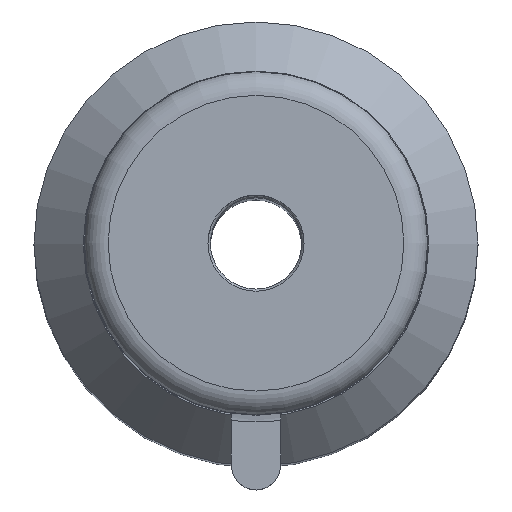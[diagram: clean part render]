
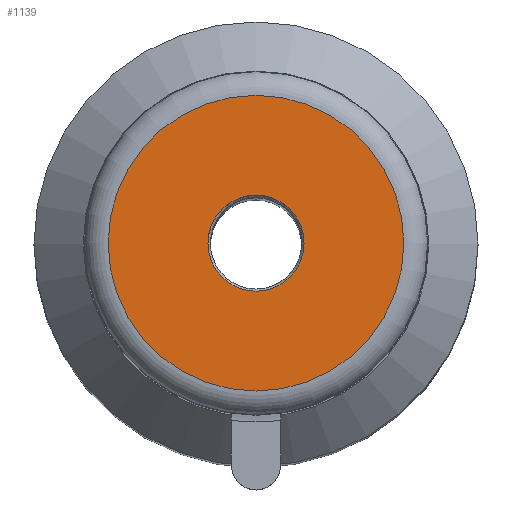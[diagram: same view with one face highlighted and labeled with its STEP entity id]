
A CAD part, top view. The second image highlights one B-rep face of the part: STEP entity #1139.
In plain terms, the highlighted planar face has unit normal (0, 0, 1).
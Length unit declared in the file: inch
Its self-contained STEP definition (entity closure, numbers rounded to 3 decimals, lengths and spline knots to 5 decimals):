
#926=CARTESIAN_POINT('',(-0.195,0.0,2.5));
#927=VERTEX_POINT('',#926);
#928=CARTESIAN_POINT('',(0.0,0.0,2.5));
#929=DIRECTION('',(0.0,0.0,-1.0));
#930=DIRECTION('',(-1.0,0.0,0.0));
#931=AXIS2_PLACEMENT_3D('',#928,#929,#930);
#932=CIRCLE('',#931,0.195);
#933=EDGE_CURVE('',#927,#927,#932,.T.);
#1014=CARTESIAN_POINT('',(-0.6,0.0,2.5));
#1015=VERTEX_POINT('',#1014);
#1016=CARTESIAN_POINT('',(0.0,0.0,2.5));
#1017=DIRECTION('',(0.0,0.0,-1.0));
#1018=DIRECTION('',(-1.0,0.0,0.0));
#1019=AXIS2_PLACEMENT_3D('',#1016,#1017,#1018);
#1020=CIRCLE('',#1019,0.6);
#1021=EDGE_CURVE('',#1015,#1015,#1020,.T.);
#1128=CARTESIAN_POINT('',(0.0,0.0,2.5));
#1129=DIRECTION('',(0.0,0.0,1.0));
#1130=DIRECTION('',(1.0,0.0,0.0));
#1131=AXIS2_PLACEMENT_3D('',#1128,#1129,#1130);
#1132=PLANE('',#1131);
#1133=ORIENTED_EDGE('',*,*,#1021,.F.);
#1134=EDGE_LOOP('',(#1133));
#1135=FACE_OUTER_BOUND('',#1134,.T.);
#1136=ORIENTED_EDGE('',*,*,#933,.T.);
#1137=EDGE_LOOP('',(#1136));
#1138=FACE_BOUND('',#1137,.T.);
#1139=ADVANCED_FACE('',(#1135,#1138),#1132,.T.);
